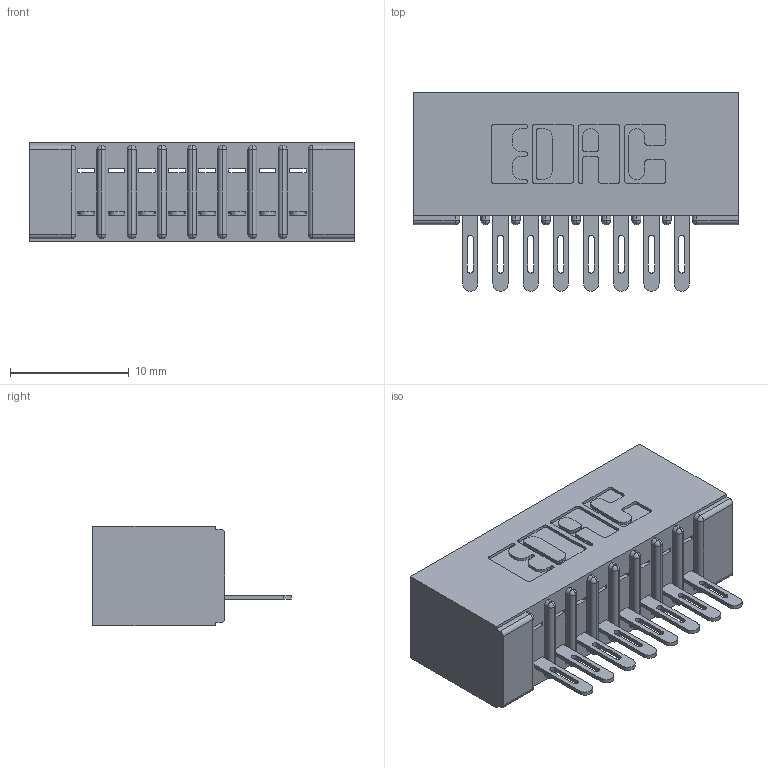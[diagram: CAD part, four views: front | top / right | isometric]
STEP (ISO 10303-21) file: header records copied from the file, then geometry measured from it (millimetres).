
FILE_DESCRIPTION (( 'STEP AP203' ), '1' );
FILE_NAME ('341-008-500-101.STEP', '2019-08-09T15:54:18', ( '' ), ( '' ), 'SwSTEP 2.0', 'SolidWorks 2016', '' );
FILE_SCHEMA (( 'CONFIG_CONTROL_DESIGN' ));
Length unit declared in the file: inch
Products named in the file (3): 341-008-500-101; 341-292-001_341-292-100; 341 Part_No Mounting Lugs
Assembly tree (9 placements, depth 2):
  341-008-500-101
    341 Part_No Mounting Lugs
    341-292-001_341-292-100  x8
Bounding box: 27.3 x 16.69 x 8.38 mm (x, y, z)
Volume: 1674.6 mm3; surface area: 2984.8 mm2
Topology: 9 solids, 9 shells, 764 faces, 2188 edges, 1406 vertices
Faces by surface type: plane 456, cylinder 276, sphere 18, torus 14
Entity records: 13685 total; most frequent: CARTESIAN_POINT 2308, ORIENTED_EDGE 2296, DIRECTION 2258, EDGE_CURVE 1148, VECTOR 890, LINE 890, VERTEX_POINT 734, AXIS2_PLACEMENT_3D 684
